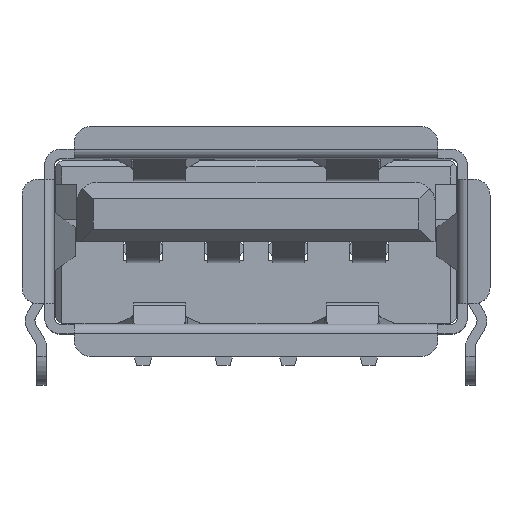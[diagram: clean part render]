
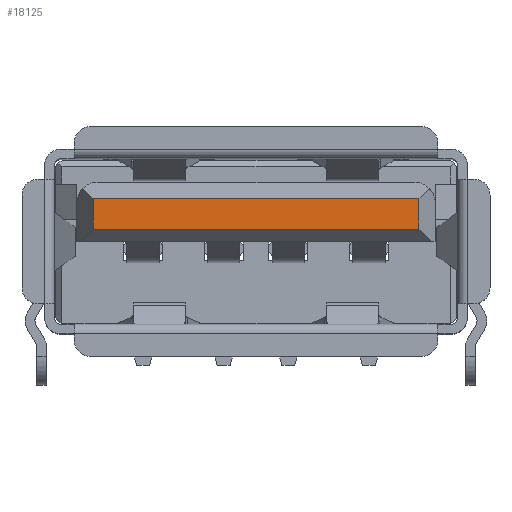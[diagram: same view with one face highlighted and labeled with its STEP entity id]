
A CAD part, top view. The second image highlights one B-rep face of the part: STEP entity #18125.
In plain terms, the highlighted face is planar.
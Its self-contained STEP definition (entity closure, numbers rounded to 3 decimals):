
#4 = EDGE_CURVE ( 'NONE', #10757, #10600, #561, .T. ) ;
#170 = CARTESIAN_POINT ( 'NONE',  ( -8.38, -1.19, 11.275 ) ) ;
#561 = LINE ( 'NONE', #6215, #11812 ) ;
#822 = VERTEX_POINT ( 'NONE', #3159 ) ;
#877 = CARTESIAN_POINT ( 'NONE',  ( -8.38, -1.19, 6.225 ) ) ;
#1319 = EDGE_CURVE ( 'NONE', #822, #5079, #12633, .T. ) ;
#1900 = ORIENTED_EDGE ( 'NONE', *, *, #5336, .F. ) ;
#2186 = VECTOR ( 'NONE', #4194, 1000. ) ;
#3151 = DIRECTION ( 'NONE',  ( 1., 0., 0. ) ) ;
#3159 = CARTESIAN_POINT ( 'NONE',  ( -8.38, -1.19, 1.175 ) ) ;
#3709 = VECTOR ( 'NONE', #18555, 1000. ) ;
#4194 = DIRECTION ( 'NONE',  ( 0., 1., 0. ) ) ;
#4480 = LINE ( 'NONE', #15155, #7464 ) ;
#5079 = VERTEX_POINT ( 'NONE', #170 ) ;
#5336 = EDGE_CURVE ( 'NONE', #5079, #10757, #4480, .T. ) ;
#5826 = ORIENTED_EDGE ( 'NONE', *, *, #4, .F. ) ;
#6215 = CARTESIAN_POINT ( 'NONE',  ( -8.38, -2.15, 6.225 ) ) ;
#7409 = ORIENTED_EDGE ( 'NONE', *, *, #1319, .F. ) ;
#7464 = VECTOR ( 'NONE', #15062, 1000. ) ;
#7721 = DIRECTION ( 'NONE',  ( 0., 0., -1. ) ) ;
#7774 = DIRECTION ( 'NONE',  ( 0., 0., -1. ) ) ;
#7988 = CARTESIAN_POINT ( 'NONE',  ( -8.38, -2.15, 11.275 ) ) ;
#8763 = CARTESIAN_POINT ( 'NONE',  ( -8.38, -1.67, 1.175 ) ) ;
#9065 = CARTESIAN_POINT ( 'NONE',  ( -8.38, -2.15, 1.175 ) ) ;
#9362 = CARTESIAN_POINT ( 'NONE',  ( -8.38, -1.67, 6.225 ) ) ;
#10536 = FACE_OUTER_BOUND ( 'NONE', #18971, .T. ) ;
#10600 = VERTEX_POINT ( 'NONE', #9065 ) ;
#10757 = VERTEX_POINT ( 'NONE', #7988 ) ;
#11812 = VECTOR ( 'NONE', #7774, 1000. ) ;
#12136 = EDGE_CURVE ( 'NONE', #10600, #822, #19047, .T. ) ;
#12139 = AXIS2_PLACEMENT_3D ( 'NONE', #9362, #3151, #7721 ) ;
#12633 = LINE ( 'NONE', #877, #3709 ) ;
#15062 = DIRECTION ( 'NONE',  ( 0., -1., 0. ) ) ;
#15155 = CARTESIAN_POINT ( 'NONE',  ( -8.38, -1.704, 11.275 ) ) ;
#16447 = PLANE ( 'NONE',  #12139 ) ;
#17920 = ORIENTED_EDGE ( 'NONE', *, *, #12136, .F. ) ;
#18125 = ADVANCED_FACE ( 'NONE', ( #10536 ), #16447, .F. ) ;
#18555 = DIRECTION ( 'NONE',  ( 0., 0., 1. ) ) ;
#18971 = EDGE_LOOP ( 'NONE', ( #7409, #17920, #5826, #1900 ) ) ;
#19047 = LINE ( 'NONE', #8763, #2186 ) ;
